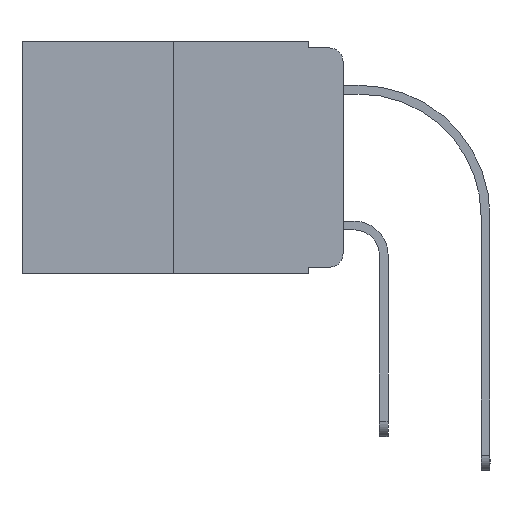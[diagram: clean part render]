
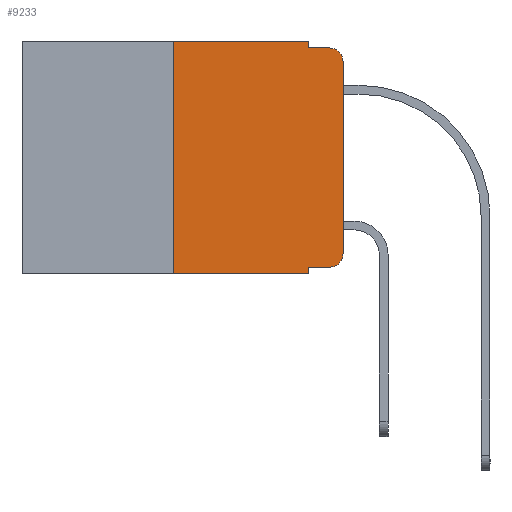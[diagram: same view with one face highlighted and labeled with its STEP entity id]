
A CAD part, left-side view. The second image highlights one B-rep face of the part: STEP entity #9233.
In plain terms, the highlighted planar face has unit normal (-1, 0, 0).
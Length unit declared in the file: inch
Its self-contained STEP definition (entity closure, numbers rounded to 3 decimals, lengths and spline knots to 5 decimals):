
#15 = VECTOR ( 'NONE', #11932, 39.37008 ) ;
#56 = ORIENTED_EDGE ( 'NONE', *, *, #10454, .T. ) ;
#63 = FACE_OUTER_BOUND ( 'NONE', #9064, .T. ) ;
#211 = VERTEX_POINT ( 'NONE', #12379 ) ;
#380 = DIRECTION ( 'NONE',  ( 0., 0., -1. ) ) ;
#845 = DIRECTION ( 'NONE',  ( 0., 0., -1. ) ) ;
#957 = VERTEX_POINT ( 'NONE', #15071 ) ;
#1181 = EDGE_CURVE ( 'NONE', #3459, #14157, #1336, .T. ) ;
#1336 = LINE ( 'NONE', #11649, #7644 ) ;
#1431 = LINE ( 'NONE', #13947, #11348 ) ;
#1715 = EDGE_CURVE ( 'NONE', #5213, #8101, #3741, .T. ) ;
#2049 = VECTOR ( 'NONE', #6684, 39.37008 ) ;
#2354 = EDGE_CURVE ( 'NONE', #211, #3459, #3179, .T. ) ;
#2562 = CARTESIAN_POINT ( 'NONE',  ( 0., 0.473, -0.343 ) ) ;
#2682 = DIRECTION ( 'NONE',  ( -1., 0., 0. ) ) ;
#2805 = VERTEX_POINT ( 'NONE', #14911 ) ;
#3122 = VERTEX_POINT ( 'NONE', #10387 ) ;
#3179 = LINE ( 'NONE', #5543, #2049 ) ;
#3459 = VERTEX_POINT ( 'NONE', #13274 ) ;
#3542 = DIRECTION ( 'NONE',  ( 0., -1., 0. ) ) ;
#3560 = CARTESIAN_POINT ( 'NONE',  ( 0., 0.473, 0. ) ) ;
#3741 = CIRCLE ( 'NONE', #5212, 0.02 ) ;
#4153 = LINE ( 'NONE', #11176, #13100 ) ;
#4925 = DIRECTION ( 'NONE',  ( 0., -1., 0. ) ) ;
#5063 = EDGE_CURVE ( 'NONE', #14157, #2805, #10785, .T. ) ;
#5212 = AXIS2_PLACEMENT_3D ( 'NONE', #13292, #2682, #14430 ) ;
#5213 = VERTEX_POINT ( 'NONE', #11178 ) ;
#5543 = CARTESIAN_POINT ( 'NONE',  ( 0., 0.25, 0. ) ) ;
#5556 = CARTESIAN_POINT ( 'NONE',  ( 0., 0.051, -0.333 ) ) ;
#5639 = CARTESIAN_POINT ( 'NONE',  ( 0., 0.051, 0. ) ) ;
#5987 = LINE ( 'NONE', #2562, #11251 ) ;
#6163 = ORIENTED_EDGE ( 'NONE', *, *, #6265, .T. ) ;
#6265 = EDGE_CURVE ( 'NONE', #957, #5213, #13390, .T. ) ;
#6684 = DIRECTION ( 'NONE',  ( 0., 0., 1. ) ) ;
#6768 = ORIENTED_EDGE ( 'NONE', *, *, #5063, .F. ) ;
#7644 = VECTOR ( 'NONE', #3542, 39.37008 ) ;
#8048 = EDGE_CURVE ( 'NONE', #211, #3122, #5987, .T. ) ;
#8101 = VERTEX_POINT ( 'NONE', #10651 ) ;
#8440 = AXIS2_PLACEMENT_3D ( 'NONE', #14637, #10978, #380 ) ;
#8465 = ORIENTED_EDGE ( 'NONE', *, *, #2354, .F. ) ;
#8579 = DIRECTION ( 'NONE',  ( 0., 0., 1. ) ) ;
#8593 = DIRECTION ( 'NONE',  ( 1., 0., 0. ) ) ;
#8800 = DIRECTION ( 'NONE',  ( 0., -1., 0. ) ) ;
#8915 = ORIENTED_EDGE ( 'NONE', *, *, #1715, .T. ) ;
#9064 = EDGE_LOOP ( 'NONE', ( #6163, #8915, #13584, #6768, #12500, #8465, #11263, #12181, #56, #13865 ) ) ;
#9233 = ADVANCED_FACE ( 'NONE', ( #63 ), #9352, .F. ) ;
#9352 = PLANE ( 'NONE',  #11622 ) ;
#9799 = EDGE_CURVE ( 'NONE', #10331, #3122, #11296, .T. ) ;
#9816 = DIRECTION ( 'NONE',  ( 0., 0., -1. ) ) ;
#10075 = EDGE_CURVE ( 'NONE', #10781, #957, #14291, .T. ) ;
#10331 = VERTEX_POINT ( 'NONE', #5556 ) ;
#10387 = CARTESIAN_POINT ( 'NONE',  ( 0., 0.051, -0.343 ) ) ;
#10454 = EDGE_CURVE ( 'NONE', #10331, #10781, #1431, .T. ) ;
#10651 = CARTESIAN_POINT ( 'NONE',  ( 0., 0.02, -0.01 ) ) ;
#10781 = VERTEX_POINT ( 'NONE', #11195 ) ;
#10785 = LINE ( 'NONE', #12014, #15 ) ;
#10859 = VECTOR ( 'NONE', #845, 39.37008 ) ;
#10978 = DIRECTION ( 'NONE',  ( -1., 0., 0. ) ) ;
#11176 = CARTESIAN_POINT ( 'NONE',  ( 0., 0.051, -0.01 ) ) ;
#11178 = CARTESIAN_POINT ( 'NONE',  ( 0., 0., -0.03 ) ) ;
#11195 = CARTESIAN_POINT ( 'NONE',  ( 0., 0.02, -0.333 ) ) ;
#11251 = VECTOR ( 'NONE', #4925, 39.37008 ) ;
#11263 = ORIENTED_EDGE ( 'NONE', *, *, #8048, .T. ) ;
#11296 = LINE ( 'NONE', #5639, #10859 ) ;
#11348 = VECTOR ( 'NONE', #13027, 39.37008 ) ;
#11622 = AXIS2_PLACEMENT_3D ( 'NONE', #3560, #8593, #9816 ) ;
#11649 = CARTESIAN_POINT ( 'NONE',  ( 0., 0.473, 0. ) ) ;
#11932 = DIRECTION ( 'NONE',  ( 0., 0., -1. ) ) ;
#12014 = CARTESIAN_POINT ( 'NONE',  ( 0., 0.051, 0. ) ) ;
#12173 = CARTESIAN_POINT ( 'NONE',  ( 0., 0., 0. ) ) ;
#12181 = ORIENTED_EDGE ( 'NONE', *, *, #9799, .F. ) ;
#12379 = CARTESIAN_POINT ( 'NONE',  ( 0., 0.25, -0.343 ) ) ;
#12496 = CARTESIAN_POINT ( 'NONE',  ( 0., 0.051, 0. ) ) ;
#12500 = ORIENTED_EDGE ( 'NONE', *, *, #1181, .F. ) ;
#13027 = DIRECTION ( 'NONE',  ( 0., -1., 0. ) ) ;
#13100 = VECTOR ( 'NONE', #8800, 39.37008 ) ;
#13274 = CARTESIAN_POINT ( 'NONE',  ( 0., 0.25, 0. ) ) ;
#13292 = CARTESIAN_POINT ( 'NONE',  ( 0., 0.02, -0.03 ) ) ;
#13390 = LINE ( 'NONE', #12173, #14647 ) ;
#13584 = ORIENTED_EDGE ( 'NONE', *, *, #14825, .F. ) ;
#13865 = ORIENTED_EDGE ( 'NONE', *, *, #10075, .T. ) ;
#13947 = CARTESIAN_POINT ( 'NONE',  ( 0., 0.051, -0.333 ) ) ;
#14157 = VERTEX_POINT ( 'NONE', #12496 ) ;
#14291 = CIRCLE ( 'NONE', #8440, 0.02 ) ;
#14430 = DIRECTION ( 'NONE',  ( 0., 0., -1. ) ) ;
#14637 = CARTESIAN_POINT ( 'NONE',  ( 0., 0.02, -0.313 ) ) ;
#14647 = VECTOR ( 'NONE', #8579, 39.37008 ) ;
#14825 = EDGE_CURVE ( 'NONE', #2805, #8101, #4153, .T. ) ;
#14911 = CARTESIAN_POINT ( 'NONE',  ( 0., 0.051, -0.01 ) ) ;
#15071 = CARTESIAN_POINT ( 'NONE',  ( 0., 0., -0.313 ) ) ;
